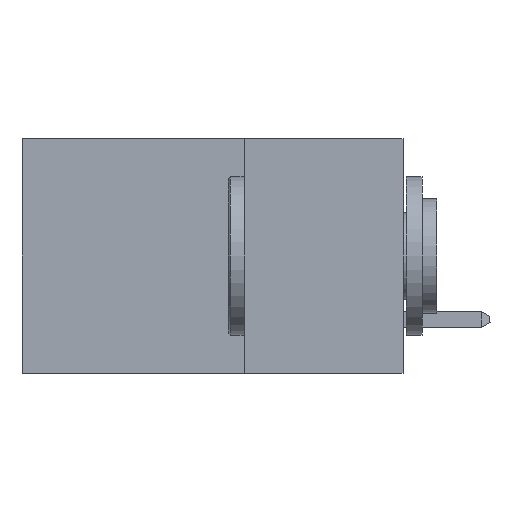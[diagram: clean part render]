
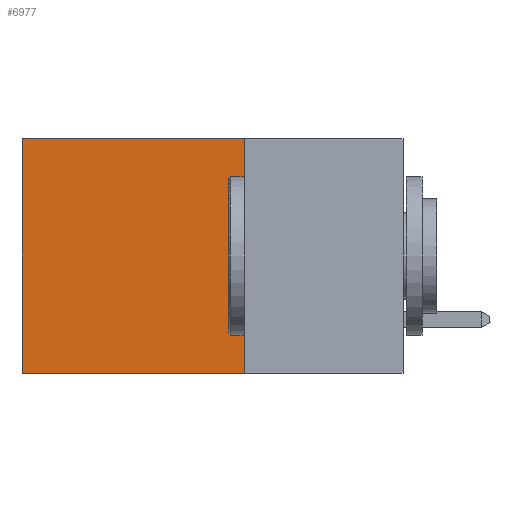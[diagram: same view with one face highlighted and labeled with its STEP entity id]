
A CAD part, left-side view. The second image highlights one B-rep face of the part: STEP entity #6977.
In plain terms, the highlighted planar face has unit normal (-1, 0, 0).
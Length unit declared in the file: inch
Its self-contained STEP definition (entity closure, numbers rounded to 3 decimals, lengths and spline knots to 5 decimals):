
#142 = LINE ( 'NONE', #2117, #3073 ) ;
#455 = VERTEX_POINT ( 'NONE', #14403 ) ;
#630 = AXIS2_PLACEMENT_3D ( 'NONE', #12564, #1851, #6234 ) ;
#1765 = VECTOR ( 'NONE', #18196, 39.37008 ) ;
#1851 = DIRECTION ( 'NONE',  ( 1., 0., 0. ) ) ;
#2117 = CARTESIAN_POINT ( 'NONE',  ( 0.2875, 0.6, 0. ) ) ;
#3073 = VECTOR ( 'NONE', #13080, 39.37008 ) ;
#3441 = EDGE_CURVE ( 'NONE', #455, #12303, #6967, .T. ) ;
#4157 = CARTESIAN_POINT ( 'NONE',  ( 0.2875, 0.25, 0. ) ) ;
#4278 = DIRECTION ( 'NONE',  ( 0., 1., 0. ) ) ;
#4954 = PLANE ( 'NONE',  #630 ) ;
#5062 = CARTESIAN_POINT ( 'NONE',  ( 0.2875, 0.6, 0. ) ) ;
#5811 = FACE_OUTER_BOUND ( 'NONE', #17647, .T. ) ;
#5819 = CARTESIAN_POINT ( 'NONE',  ( 0.2875, 0.6, -0.37 ) ) ;
#6234 = DIRECTION ( 'NONE',  ( 0., 0., -1. ) ) ;
#6245 = EDGE_CURVE ( 'NONE', #12303, #13525, #13312, .T. ) ;
#6967 = LINE ( 'NONE', #16089, #19688 ) ;
#6977 = ADVANCED_FACE ( 'NONE', ( #5811 ), #4954, .F. ) ;
#7084 = ORIENTED_EDGE ( 'NONE', *, *, #12016, .T. ) ;
#8512 = DIRECTION ( 'NONE',  ( 0., 0., -1. ) ) ;
#9251 = LINE ( 'NONE', #4157, #10704 ) ;
#10704 = VECTOR ( 'NONE', #4278, 39.37008 ) ;
#12016 = EDGE_CURVE ( 'NONE', #455, #12785, #9251, .T. ) ;
#12303 = VERTEX_POINT ( 'NONE', #17193 ) ;
#12564 = CARTESIAN_POINT ( 'NONE',  ( 0.2875, 0.25, 0. ) ) ;
#12785 = VERTEX_POINT ( 'NONE', #5062 ) ;
#13080 = DIRECTION ( 'NONE',  ( 0., 0., -1. ) ) ;
#13312 = LINE ( 'NONE', #16322, #1765 ) ;
#13525 = VERTEX_POINT ( 'NONE', #5819 ) ;
#13831 = EDGE_CURVE ( 'NONE', #12785, #13525, #142, .T. ) ;
#14403 = CARTESIAN_POINT ( 'NONE',  ( 0.2875, 0.25, 0. ) ) ;
#15242 = ORIENTED_EDGE ( 'NONE', *, *, #13831, .T. ) ;
#15884 = ORIENTED_EDGE ( 'NONE', *, *, #3441, .F. ) ;
#16089 = CARTESIAN_POINT ( 'NONE',  ( 0.2875, 0.25, 0. ) ) ;
#16322 = CARTESIAN_POINT ( 'NONE',  ( 0.2875, 0.25, -0.37 ) ) ;
#16547 = ORIENTED_EDGE ( 'NONE', *, *, #6245, .F. ) ;
#17193 = CARTESIAN_POINT ( 'NONE',  ( 0.2875, 0.25, -0.37 ) ) ;
#17647 = EDGE_LOOP ( 'NONE', ( #15242, #16547, #15884, #7084 ) ) ;
#18196 = DIRECTION ( 'NONE',  ( 0., 1., 0. ) ) ;
#19688 = VECTOR ( 'NONE', #8512, 39.37008 ) ;
